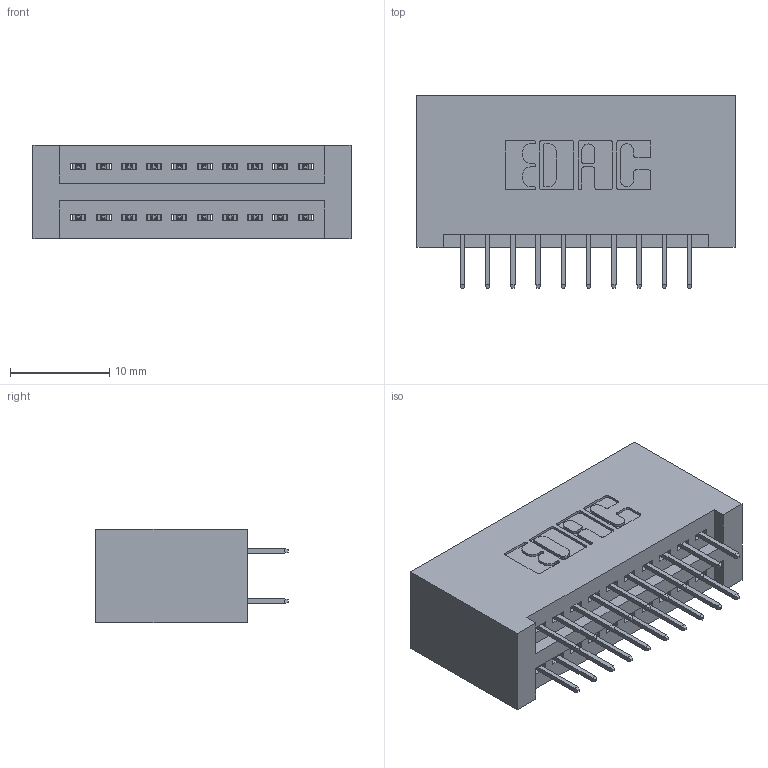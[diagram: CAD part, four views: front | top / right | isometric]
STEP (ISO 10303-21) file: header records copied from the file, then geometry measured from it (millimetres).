
FILE_DESCRIPTION (( 'STEP AP203' ), '1' );
FILE_NAME ('395-020-524-201.STEP', '2019-10-15T21:04:05', ( '' ), ( '' ), 'SwSTEP 2.0', 'SolidWorks 2016', '' );
FILE_SCHEMA (( 'CONFIG_CONTROL_DESIGN' ));
Length unit declared in the file: inch
Products named in the file (3): 345 Part_No Mounting Lugs; 345-292-001_345-293-124; 395-020-524-201
Assembly tree (21 placements, depth 2):
  395-020-524-201
    345 Part_No Mounting Lugs
    345-292-001_345-293-124  x20
Bounding box: 32 x 19.35 x 9.4 mm (x, y, z)
Volume: 3397.5 mm3; surface area: 4625.7 mm2
Topology: 21 solids, 21 shells, 1198 faces, 3377 edges, 2170 vertices
Faces by surface type: plane 856, cylinder 342
Entity records: 11951 total; most frequent: CARTESIAN_POINT 2032, ORIENTED_EDGE 1966, DIRECTION 1827, EDGE_CURVE 983, LINE 823, VECTOR 823, VERTEX_POINT 650, AXIS2_PLACEMENT_3D 502
